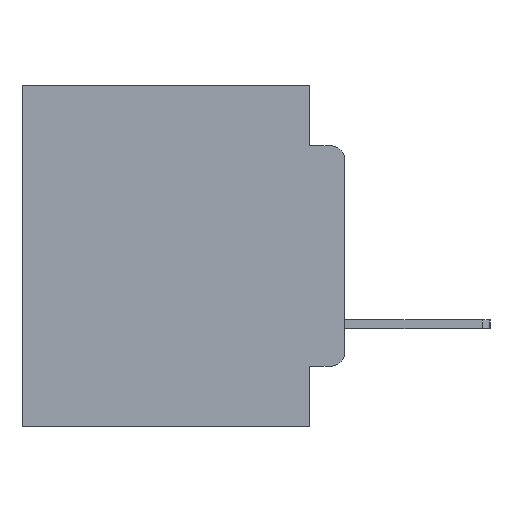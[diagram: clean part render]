
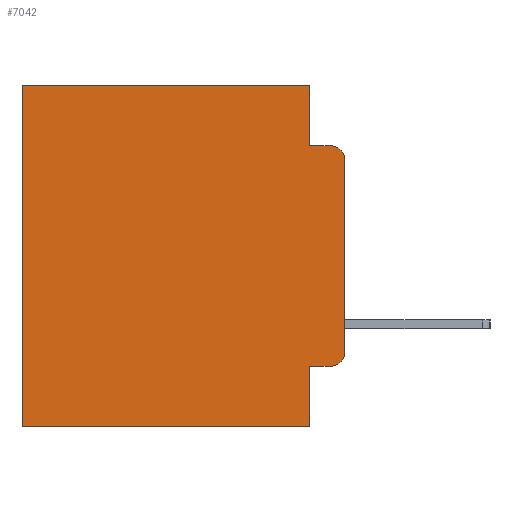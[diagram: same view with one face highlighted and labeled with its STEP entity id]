
A CAD part, left-side view. The second image highlights one B-rep face of the part: STEP entity #7042.
In plain terms, the highlighted planar face has unit normal (-1, 0, 0).
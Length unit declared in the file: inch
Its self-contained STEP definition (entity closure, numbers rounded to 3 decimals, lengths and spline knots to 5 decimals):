
#380 = EDGE_CURVE ( 'NONE', #4555, #5146, #16570, .T. ) ;
#840 = EDGE_LOOP ( 'NONE', ( #8227, #11669, #4058, #20172, #14632, #5313, #20741, #23012, #19351, #21880 ) ) ;
#1022 = EDGE_CURVE ( 'NONE', #4555, #16748, #17751, .T. ) ;
#2074 = LINE ( 'NONE', #3909, #17241 ) ;
#2109 = CARTESIAN_POINT ( 'NONE',  ( 0.298, 0.051, 0. ) ) ;
#2876 = LINE ( 'NONE', #7094, #7728 ) ;
#3284 = EDGE_CURVE ( 'NONE', #16748, #4731, #16574, .T. ) ;
#3909 = CARTESIAN_POINT ( 'NONE',  ( 0.298, 0.051, -0.0885 ) ) ;
#4058 = ORIENTED_EDGE ( 'NONE', *, *, #21924, .F. ) ;
#4400 = DIRECTION ( 'NONE',  ( -1., 0., 0. ) ) ;
#4555 = VERTEX_POINT ( 'NONE', #19741 ) ;
#4731 = VERTEX_POINT ( 'NONE', #15788 ) ;
#4932 = DIRECTION ( 'NONE',  ( 0., 1., 0. ) ) ;
#4938 = CARTESIAN_POINT ( 'NONE',  ( 0.298, 0., 0. ) ) ;
#5146 = VERTEX_POINT ( 'NONE', #11861 ) ;
#5313 = ORIENTED_EDGE ( 'NONE', *, *, #3284, .T. ) ;
#5981 = AXIS2_PLACEMENT_3D ( 'NONE', #4938, #14831, #9098 ) ;
#6003 = VECTOR ( 'NONE', #4932, 39.37008 ) ;
#6237 = CARTESIAN_POINT ( 'NONE',  ( 0.298, 0.051, -0.4115 ) ) ;
#6333 = CIRCLE ( 'NONE', #13276, 0.02 ) ;
#6360 = DIRECTION ( 'NONE',  ( 0., -1., 0. ) ) ;
#6993 = PLANE ( 'NONE',  #5981 ) ;
#7042 = ADVANCED_FACE ( 'NONE', ( #8602 ), #6993, .F. ) ;
#7094 = CARTESIAN_POINT ( 'NONE',  ( 0.298, 0., 0. ) ) ;
#7140 = VERTEX_POINT ( 'NONE', #13182 ) ;
#7401 = EDGE_CURVE ( 'NONE', #7824, #10538, #19102, .T. ) ;
#7728 = VECTOR ( 'NONE', #13106, 39.37008 ) ;
#7824 = VERTEX_POINT ( 'NONE', #6237 ) ;
#8227 = ORIENTED_EDGE ( 'NONE', *, *, #15703, .F. ) ;
#8602 = FACE_OUTER_BOUND ( 'NONE', #840, .T. ) ;
#8732 = LINE ( 'NONE', #23430, #23147 ) ;
#8794 = EDGE_CURVE ( 'NONE', #7824, #19204, #8732, .T. ) ;
#9049 = VERTEX_POINT ( 'NONE', #19025 ) ;
#9098 = DIRECTION ( 'NONE',  ( 0., 0., -1. ) ) ;
#10074 = DIRECTION ( 'NONE',  ( 0., 0., -1. ) ) ;
#10135 = CARTESIAN_POINT ( 'NONE',  ( 0.298, 0.473, 0. ) ) ;
#10538 = VERTEX_POINT ( 'NONE', #19287 ) ;
#11418 = LINE ( 'NONE', #16665, #6003 ) ;
#11489 = EDGE_CURVE ( 'NONE', #19204, #9049, #6333, .T. ) ;
#11620 = VECTOR ( 'NONE', #10074, 39.37008 ) ;
#11669 = ORIENTED_EDGE ( 'NONE', *, *, #19519, .T. ) ;
#11797 = EDGE_CURVE ( 'NONE', #10538, #4731, #11418, .T. ) ;
#11861 = CARTESIAN_POINT ( 'NONE',  ( 0.298, 0.051, -0.0885 ) ) ;
#12072 = CARTESIAN_POINT ( 'NONE',  ( 0.298, 0.02, -0.3915 ) ) ;
#12193 = VECTOR ( 'NONE', #20556, 39.37008 ) ;
#13106 = DIRECTION ( 'NONE',  ( 0., 0., -1. ) ) ;
#13182 = CARTESIAN_POINT ( 'NONE',  ( 0.298, 0.02, -0.0885 ) ) ;
#13276 = AXIS2_PLACEMENT_3D ( 'NONE', #12072, #25024, #13999 ) ;
#13960 = VECTOR ( 'NONE', #21422, 39.37008 ) ;
#13999 = DIRECTION ( 'NONE',  ( 0., 0., -1. ) ) ;
#14178 = DIRECTION ( 'NONE',  ( 0., 0., -1. ) ) ;
#14632 = ORIENTED_EDGE ( 'NONE', *, *, #1022, .T. ) ;
#14831 = DIRECTION ( 'NONE',  ( 1., 0., 0. ) ) ;
#15573 = AXIS2_PLACEMENT_3D ( 'NONE', #16163, #4400, #18092 ) ;
#15703 = EDGE_CURVE ( 'NONE', #18026, #9049, #2876, .T. ) ;
#15788 = CARTESIAN_POINT ( 'NONE',  ( 0.298, 0.473, -0.5 ) ) ;
#16163 = CARTESIAN_POINT ( 'NONE',  ( 0.298, 0.02, -0.1085 ) ) ;
#16570 = LINE ( 'NONE', #18963, #11620 ) ;
#16574 = LINE ( 'NONE', #20654, #12193 ) ;
#16665 = CARTESIAN_POINT ( 'NONE',  ( 0.298, 0., -0.5 ) ) ;
#16748 = VERTEX_POINT ( 'NONE', #10135 ) ;
#17241 = VECTOR ( 'NONE', #17628, 39.37008 ) ;
#17628 = DIRECTION ( 'NONE',  ( 0., -1., 0. ) ) ;
#17751 = LINE ( 'NONE', #23585, #13960 ) ;
#18026 = VERTEX_POINT ( 'NONE', #18791 ) ;
#18092 = DIRECTION ( 'NONE',  ( 0., 0., -1. ) ) ;
#18791 = CARTESIAN_POINT ( 'NONE',  ( 0.298, 0., -0.1085 ) ) ;
#18963 = CARTESIAN_POINT ( 'NONE',  ( 0.298, 0.051, 0. ) ) ;
#19025 = CARTESIAN_POINT ( 'NONE',  ( 0.298, 0., -0.3915 ) ) ;
#19102 = LINE ( 'NONE', #2109, #23910 ) ;
#19204 = VERTEX_POINT ( 'NONE', #23211 ) ;
#19287 = CARTESIAN_POINT ( 'NONE',  ( 0.298, 0.051, -0.5 ) ) ;
#19351 = ORIENTED_EDGE ( 'NONE', *, *, #8794, .T. ) ;
#19519 = EDGE_CURVE ( 'NONE', #18026, #7140, #20683, .T. ) ;
#19741 = CARTESIAN_POINT ( 'NONE',  ( 0.298, 0.051, 0. ) ) ;
#20172 = ORIENTED_EDGE ( 'NONE', *, *, #380, .F. ) ;
#20556 = DIRECTION ( 'NONE',  ( 0., 0., -1. ) ) ;
#20654 = CARTESIAN_POINT ( 'NONE',  ( 0.298, 0.473, 0. ) ) ;
#20683 = CIRCLE ( 'NONE', #15573, 0.02 ) ;
#20741 = ORIENTED_EDGE ( 'NONE', *, *, #11797, .F. ) ;
#21422 = DIRECTION ( 'NONE',  ( 0., 1., 0. ) ) ;
#21880 = ORIENTED_EDGE ( 'NONE', *, *, #11489, .T. ) ;
#21924 = EDGE_CURVE ( 'NONE', #5146, #7140, #2074, .T. ) ;
#23012 = ORIENTED_EDGE ( 'NONE', *, *, #7401, .F. ) ;
#23147 = VECTOR ( 'NONE', #6360, 39.37008 ) ;
#23211 = CARTESIAN_POINT ( 'NONE',  ( 0.298, 0.02, -0.4115 ) ) ;
#23430 = CARTESIAN_POINT ( 'NONE',  ( 0.298, 0.051, -0.4115 ) ) ;
#23585 = CARTESIAN_POINT ( 'NONE',  ( 0.298, 0., 0. ) ) ;
#23910 = VECTOR ( 'NONE', #14178, 39.37008 ) ;
#25024 = DIRECTION ( 'NONE',  ( -1., 0., 0. ) ) ;
